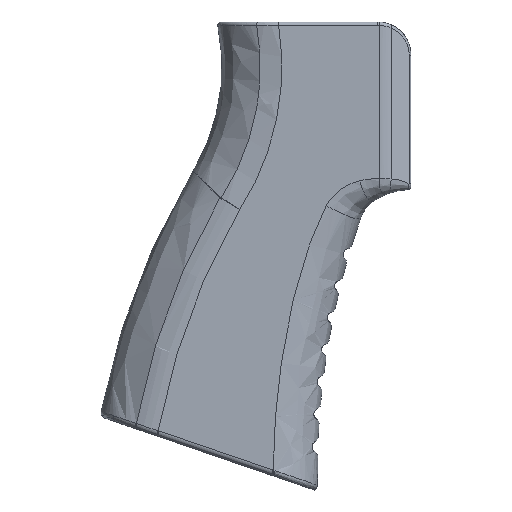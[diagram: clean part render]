
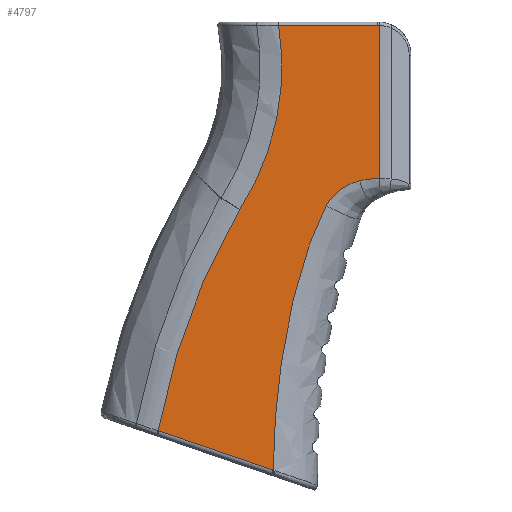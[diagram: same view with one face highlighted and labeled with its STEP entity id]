
A CAD part, left-side view. The second image highlights one B-rep face of the part: STEP entity #4797.
In plain terms, the highlighted planar face has unit normal (-1, 0, 0).
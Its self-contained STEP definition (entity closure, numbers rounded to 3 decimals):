
#70=PLANE('',#5243);
#187=B_SPLINE_CURVE_WITH_KNOTS('',3,(#8496,#8497,#8498,#8499),
 .UNSPECIFIED.,.F.,.F.,(4,4),(0.,0.009),
 .UNSPECIFIED.);
#195=B_SPLINE_CURVE_WITH_KNOTS('',3,(#8601,#8602,#8603,#8604),
 .UNSPECIFIED.,.F.,.F.,(4,4),(0.,0.007),
 .UNSPECIFIED.);
#244=B_SPLINE_CURVE_WITH_KNOTS('',3,(#9635,#9636,#9637,#9638),
 .UNSPECIFIED.,.F.,.F.,(4,4),(-4.543,-0.013),
 .UNSPECIFIED.);
#248=B_SPLINE_CURVE_WITH_KNOTS('',3,(#9657,#9658,#9659,#9660,#9661,#9662,
#9663),.UNSPECIFIED.,.F.,.F.,(4,1,1,1,4),(-6.152,-5.367,
-4.581,-3.01,-0.953),.UNSPECIFIED.);
#249=B_SPLINE_CURVE_WITH_KNOTS('',3,(#9665,#9666,#9667,#9668,#9669,#9670,
#9671),.UNSPECIFIED.,.F.,.F.,(4,1,1,1,4),(-7.01,-7.008,
-6.58,-6.366,-6.152),.UNSPECIFIED.);
#250=B_SPLINE_CURVE_WITH_KNOTS('',3,(#9673,#9674,#9675,#9676,#9677,#9678,
#9679,#9680,#9681,#9682,#9683,#9684,#9685,#9686,#9687,#9688,#9689,#9690,
#9691,#9692),.UNSPECIFIED.,.F.,.F.,(4,1,1,1,1,1,1,1,1,1,1,1,1,1,1,1,1,4),
(-7.396,-7.394,-7.377,-7.36,
-7.268,-7.219,-7.196,-7.18,-7.165,
-7.149,-7.134,-7.118,-7.087,
-7.071,-7.055,-7.04,-7.024,
-7.01),.UNSPECIFIED.);
#251=B_SPLINE_CURVE_WITH_KNOTS('',3,(#9694,#9695,#9696,#9697,#9698),
 .UNSPECIFIED.,.F.,.F.,(4,1,4),(-7.41,-7.407,-7.396),
 .UNSPECIFIED.);
#252=B_SPLINE_CURVE_WITH_KNOTS('',3,(#9706,#9707,#9708,#9709,#9710),
 .UNSPECIFIED.,.F.,.F.,(4,1,4),(-1.958,-1.682,-0.143),
 .UNSPECIFIED.);
#253=B_SPLINE_CURVE_WITH_KNOTS('',3,(#9711,#9712,#9713,#9714),
 .UNSPECIFIED.,.F.,.F.,(4,4),(-3.822,-1.958),
 .UNSPECIFIED.);
#750=FACE_OUTER_BOUND('',#1053,.T.);
#1053=EDGE_LOOP('',(#3766,#3767,#3768,#3769,#3770,#3771,#3772,#3773,#3774,
#3775,#3776,#3777,#3778));
#1259=LINE('',#8469,#1427);
#1276=LINE('',#9700,#1444);
#1277=LINE('',#9704,#1445);
#1427=VECTOR('',#5985,10.);
#1444=VECTOR('',#6052,10.);
#1445=VECTOR('',#6055,10.);
#1712=CIRCLE('',#5244,5.71);
#1984=VERTEX_POINT('',#8466);
#1985=VERTEX_POINT('',#8468);
#1987=VERTEX_POINT('',#8489);
#1992=VERTEX_POINT('',#8548);
#2051=VERTEX_POINT('',#9634);
#2054=VERTEX_POINT('',#9656);
#2055=VERTEX_POINT('',#9664);
#2056=VERTEX_POINT('',#9672);
#2057=VERTEX_POINT('',#9693);
#2058=VERTEX_POINT('',#9699);
#2059=VERTEX_POINT('',#9701);
#2060=VERTEX_POINT('',#9703);
#2061=VERTEX_POINT('',#9705);
#2580=EDGE_CURVE('',#1984,#1985,#1259,.T.);
#2585=EDGE_CURVE('',#1985,#1987,#187,.T.);
#2596=EDGE_CURVE('',#1987,#1992,#195,.T.);
#2680=EDGE_CURVE('',#1992,#2051,#244,.T.);
#2684=EDGE_CURVE('',#2054,#1984,#248,.T.);
#2685=EDGE_CURVE('',#2055,#2054,#249,.T.);
#2686=EDGE_CURVE('',#2056,#2055,#250,.T.);
#2687=EDGE_CURVE('',#2057,#2056,#251,.T.);
#2688=EDGE_CURVE('',#2058,#2057,#1276,.T.);
#2689=EDGE_CURVE('',#2059,#2058,#1712,.T.);
#2690=EDGE_CURVE('',#2060,#2059,#1277,.T.);
#2691=EDGE_CURVE('',#2061,#2060,#252,.T.);
#2692=EDGE_CURVE('',#2051,#2061,#253,.T.);
#3766=ORIENTED_EDGE('',*,*,#2596,.F.);
#3767=ORIENTED_EDGE('',*,*,#2585,.F.);
#3768=ORIENTED_EDGE('',*,*,#2580,.F.);
#3769=ORIENTED_EDGE('',*,*,#2684,.F.);
#3770=ORIENTED_EDGE('',*,*,#2685,.F.);
#3771=ORIENTED_EDGE('',*,*,#2686,.F.);
#3772=ORIENTED_EDGE('',*,*,#2687,.F.);
#3773=ORIENTED_EDGE('',*,*,#2688,.F.);
#3774=ORIENTED_EDGE('',*,*,#2689,.F.);
#3775=ORIENTED_EDGE('',*,*,#2690,.F.);
#3776=ORIENTED_EDGE('',*,*,#2691,.F.);
#3777=ORIENTED_EDGE('',*,*,#2692,.F.);
#3778=ORIENTED_EDGE('',*,*,#2680,.F.);
#4797=ADVANCED_FACE('',(#750),#70,.T.);
#5243=AXIS2_PLACEMENT_3D('',#9655,#6050,#6051);
#5244=AXIS2_PLACEMENT_3D('',#9702,#6053,#6054);
#5985=DIRECTION('',(0.,0.946,0.324));
#6050=DIRECTION('center_axis',(-1.,0.,0.));
#6051=DIRECTION('ref_axis',(0.,-1.,0.));
#6052=DIRECTION('',(0.,0.,-1.));
#6053=DIRECTION('center_axis',(1.,0.,0.));
#6054=DIRECTION('ref_axis',(0.,-0.022,1.));
#6055=DIRECTION('',(0.,-1.,0.));
#8466=CARTESIAN_POINT('',(12.918,-123.483,-57.259));
#8468=CARTESIAN_POINT('',(12.918,-101.663,-49.787));
#8469=CARTESIAN_POINT('',(12.918,-3.74,-16.258));
#8489=CARTESIAN_POINT('',(12.918,-101.578,-49.758));
#8496=CARTESIAN_POINT('Ctrl Pts',(12.918,-101.663,-49.787));
#8497=CARTESIAN_POINT('Ctrl Pts',(12.918,-101.634,-49.778));
#8498=CARTESIAN_POINT('Ctrl Pts',(12.918,-101.606,-49.768));
#8499=CARTESIAN_POINT('Ctrl Pts',(12.918,-101.578,-49.758));
#8548=CARTESIAN_POINT('',(12.918,-101.512,-49.735));
#8601=CARTESIAN_POINT('Ctrl Pts',(12.918,-101.578,-49.758));
#8602=CARTESIAN_POINT('Ctrl Pts',(12.918,-101.556,-49.75));
#8603=CARTESIAN_POINT('Ctrl Pts',(12.918,-101.534,-49.743));
#8604=CARTESIAN_POINT('Ctrl Pts',(12.918,-101.512,-49.735));
#9634=CARTESIAN_POINT('',(12.918,-117.077,-7.435));
#9635=CARTESIAN_POINT('Ctrl Pts',(12.918,-101.512,-49.735));
#9636=CARTESIAN_POINT('Ctrl Pts',(12.918,-104.188,-34.873));
#9637=CARTESIAN_POINT('Ctrl Pts',(12.918,-109.481,-20.487));
#9638=CARTESIAN_POINT('Ctrl Pts',(12.918,-117.077,-7.435));
#9655=CARTESIAN_POINT('Origin',(12.918,31.889,-6.377));
#9656=CARTESIAN_POINT('',(12.918,-133.636,-6.732));
#9657=CARTESIAN_POINT('Ctrl Pts',(12.918,-133.636,-6.732));
#9658=CARTESIAN_POINT('Ctrl Pts',(12.918,-132.386,-8.991));
#9659=CARTESIAN_POINT('Ctrl Pts',(12.918,-130.396,-13.842));
#9660=CARTESIAN_POINT('Ctrl Pts',(12.918,-127.298,-23.844));
#9661=CARTESIAN_POINT('Ctrl Pts',(12.918,-124.454,-38.313));
#9662=CARTESIAN_POINT('Ctrl Pts',(12.918,-123.548,-50.4));
#9663=CARTESIAN_POINT('Ctrl Pts',(12.918,-123.483,-57.259));
#9664=CARTESIAN_POINT('',(12.918,-140.048,-1.924));
#9665=CARTESIAN_POINT('Ctrl Pts',(12.918,-140.048,-1.924));
#9666=CARTESIAN_POINT('Ctrl Pts',(12.918,-140.042,-1.925));
#9667=CARTESIAN_POINT('Ctrl Pts',(12.918,-138.732,-2.236));
#9668=CARTESIAN_POINT('Ctrl Pts',(12.918,-136.844,-3.101));
#9669=CARTESIAN_POINT('Ctrl Pts',(12.918,-134.788,-4.965));
#9670=CARTESIAN_POINT('Ctrl Pts',(12.918,-133.976,-6.116));
#9671=CARTESIAN_POINT('Ctrl Pts',(12.918,-133.636,-6.732));
#9672=CARTESIAN_POINT('',(12.918,-143.606,-1.546));
#9673=CARTESIAN_POINT('Ctrl Pts',(12.918,-143.606,-1.546));
#9674=CARTESIAN_POINT('Ctrl Pts',(12.918,-143.6,-1.546));
#9675=CARTESIAN_POINT('Ctrl Pts',(12.918,-143.544,-1.545));
#9676=CARTESIAN_POINT('Ctrl Pts',(12.918,-143.435,-1.543));
#9677=CARTESIAN_POINT('Ctrl Pts',(12.918,-143.049,-1.542));
#9678=CARTESIAN_POINT('Ctrl Pts',(12.918,-142.563,-1.557));
#9679=CARTESIAN_POINT('Ctrl Pts',(12.918,-142.053,-1.598));
#9680=CARTESIAN_POINT('Ctrl Pts',(12.918,-141.781,-1.626));
#9681=CARTESIAN_POINT('Ctrl Pts',(12.918,-141.613,-1.645));
#9682=CARTESIAN_POINT('Ctrl Pts',(12.918,-141.469,-1.663));
#9683=CARTESIAN_POINT('Ctrl Pts',(12.918,-141.326,-1.683));
#9684=CARTESIAN_POINT('Ctrl Pts',(12.918,-141.182,-1.704));
#9685=CARTESIAN_POINT('Ctrl Pts',(12.918,-140.99,-1.734));
#9686=CARTESIAN_POINT('Ctrl Pts',(12.918,-140.798,-1.767));
#9687=CARTESIAN_POINT('Ctrl Pts',(12.918,-140.606,-1.803));
#9688=CARTESIAN_POINT('Ctrl Pts',(12.918,-140.462,-1.832));
#9689=CARTESIAN_POINT('Ctrl Pts',(12.918,-140.318,-1.863));
#9690=CARTESIAN_POINT('Ctrl Pts',(12.918,-140.18,-1.893));
#9691=CARTESIAN_POINT('Ctrl Pts',(12.918,-140.09,-1.914));
#9692=CARTESIAN_POINT('Ctrl Pts',(12.918,-140.048,-1.924));
#9693=CARTESIAN_POINT('',(12.918,-143.742,-1.549));
#9694=CARTESIAN_POINT('Ctrl Pts',(12.918,-143.742,-1.549));
#9695=CARTESIAN_POINT('Ctrl Pts',(12.918,-143.731,-1.549));
#9696=CARTESIAN_POINT('Ctrl Pts',(12.918,-143.686,-1.548));
#9697=CARTESIAN_POINT('Ctrl Pts',(12.918,-143.641,-1.547));
#9698=CARTESIAN_POINT('Ctrl Pts',(12.918,-143.606,-1.546));
#9699=CARTESIAN_POINT('',(12.918,-143.742,27.759));
#9700=CARTESIAN_POINT('',(12.918,-143.742,11.014));
#9701=CARTESIAN_POINT('',(12.918,-143.468,27.766));
#9702=CARTESIAN_POINT('Origin',(12.918,-143.468,22.056));
#9703=CARTESIAN_POINT('',(12.918,-124.522,27.766));
#9704=CARTESIAN_POINT('',(12.918,-40.367,27.766));
#9705=CARTESIAN_POINT('',(12.918,-124.104,9.713));
#9706=CARTESIAN_POINT('Ctrl Pts',(12.918,-124.103,9.714));
#9707=CARTESIAN_POINT('Ctrl Pts',(12.918,-124.29,10.615));
#9708=CARTESIAN_POINT('Ctrl Pts',(12.918,-125.355,16.574));
#9709=CARTESIAN_POINT('Ctrl Pts',(12.918,-125.326,22.698));
#9710=CARTESIAN_POINT('Ctrl Pts',(12.918,-124.522,27.766));
#9711=CARTESIAN_POINT('Ctrl Pts',(12.918,-117.077,-7.435));
#9712=CARTESIAN_POINT('Ctrl Pts',(12.918,-120.451,-2.219));
#9713=CARTESIAN_POINT('Ctrl Pts',(12.918,-122.843,3.631));
#9714=CARTESIAN_POINT('Ctrl Pts',(12.918,-124.103,9.714));
